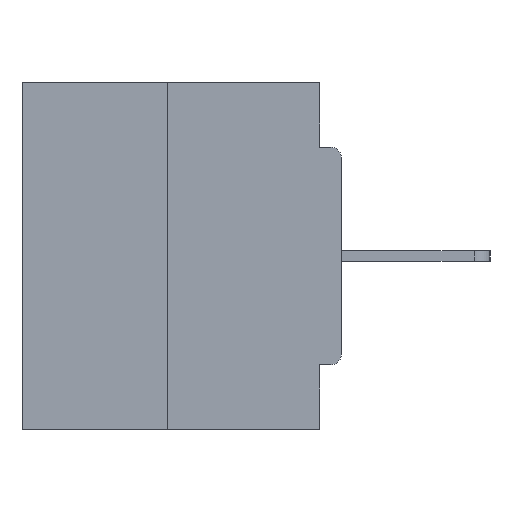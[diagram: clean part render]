
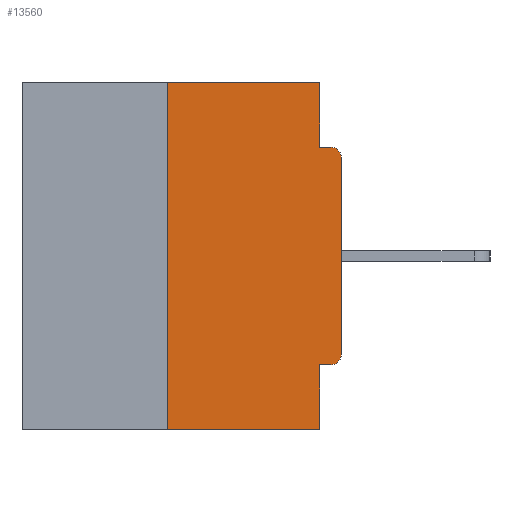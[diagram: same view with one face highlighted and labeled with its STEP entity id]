
A CAD part, left-side view. The second image highlights one B-rep face of the part: STEP entity #13560.
In plain terms, the highlighted planar face has unit normal (-1, 0, 0).
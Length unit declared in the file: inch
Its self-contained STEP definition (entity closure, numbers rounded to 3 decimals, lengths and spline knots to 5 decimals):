
#351 = EDGE_CURVE ( 'NONE', #19946, #1545, #28902, .T. ) ;
#399 = AXIS2_PLACEMENT_3D ( 'NONE', #8657, #17808, #10980 ) ;
#651 = LINE ( 'NONE', #26671, #6100 ) ;
#887 = VECTOR ( 'NONE', #17374, 39.37008 ) ;
#1545 = VERTEX_POINT ( 'NONE', #16060 ) ;
#1696 = AXIS2_PLACEMENT_3D ( 'NONE', #14558, #9563, #14642 ) ;
#1831 = VERTEX_POINT ( 'NONE', #20612 ) ;
#1855 = VERTEX_POINT ( 'NONE', #7345 ) ;
#2134 = CARTESIAN_POINT ( 'NONE',  ( 0., 0.46, 0. ) ) ;
#2260 = ORIENTED_EDGE ( 'NONE', *, *, #26404, .F. ) ;
#2754 = CIRCLE ( 'NONE', #399, 0.015 ) ;
#2787 = VERTEX_POINT ( 'NONE', #12997 ) ;
#3079 = LINE ( 'NONE', #26126, #11424 ) ;
#3674 = DIRECTION ( 'NONE',  ( 0., 0., -1. ) ) ;
#4083 = EDGE_CURVE ( 'NONE', #1855, #2787, #651, .T. ) ;
#4960 = VECTOR ( 'NONE', #9685, 39.37008 ) ;
#5619 = EDGE_CURVE ( 'NONE', #1831, #19946, #8171, .T. ) ;
#5686 = CARTESIAN_POINT ( 'NONE',  ( 0., 0.015, -0.0935 ) ) ;
#6100 = VECTOR ( 'NONE', #24642, 39.37008 ) ;
#6705 = LINE ( 'NONE', #8227, #27568 ) ;
#7345 = CARTESIAN_POINT ( 'NONE',  ( 0., 0., -0.3915 ) ) ;
#7649 = DIRECTION ( 'NONE',  ( 0., 0., -1. ) ) ;
#7907 = VERTEX_POINT ( 'NONE', #17746 ) ;
#7936 = AXIS2_PLACEMENT_3D ( 'NONE', #21834, #8075, #17742 ) ;
#8075 = DIRECTION ( 'NONE',  ( -1., 0., 0. ) ) ;
#8171 = LINE ( 'NONE', #25965, #4960 ) ;
#8227 = CARTESIAN_POINT ( 'NONE',  ( 0., 0.031, 0. ) ) ;
#8627 = ORIENTED_EDGE ( 'NONE', *, *, #17073, .T. ) ;
#8657 = CARTESIAN_POINT ( 'NONE',  ( 0., 0.015, -0.3915 ) ) ;
#9251 = LINE ( 'NONE', #20959, #17559 ) ;
#9563 = DIRECTION ( 'NONE',  ( 1., 0., 0. ) ) ;
#9685 = DIRECTION ( 'NONE',  ( 0., 0., 1. ) ) ;
#10751 = CARTESIAN_POINT ( 'NONE',  ( 0., 0., -0.0935 ) ) ;
#10980 = DIRECTION ( 'NONE',  ( 0., 0., -1. ) ) ;
#11026 = VERTEX_POINT ( 'NONE', #22522 ) ;
#11259 = ORIENTED_EDGE ( 'NONE', *, *, #15847, .T. ) ;
#11424 = VECTOR ( 'NONE', #7649, 39.37008 ) ;
#12436 = CARTESIAN_POINT ( 'NONE',  ( 0., 0.25, 0. ) ) ;
#12734 = EDGE_CURVE ( 'NONE', #22730, #25406, #3079, .T. ) ;
#12776 = CIRCLE ( 'NONE', #7936, 0.015 ) ;
#12997 = CARTESIAN_POINT ( 'NONE',  ( 0., 0., -0.1085 ) ) ;
#13276 = CARTESIAN_POINT ( 'NONE',  ( 0., 0.46, -0.5 ) ) ;
#13560 = ADVANCED_FACE ( 'NONE', ( #21498 ), #23352, .F. ) ;
#13973 = LINE ( 'NONE', #10751, #887 ) ;
#14558 = CARTESIAN_POINT ( 'NONE',  ( 0., 0.46, 0. ) ) ;
#14642 = DIRECTION ( 'NONE',  ( 0., 0., -1. ) ) ;
#15584 = ORIENTED_EDGE ( 'NONE', *, *, #16656, .F. ) ;
#15629 = VECTOR ( 'NONE', #20838, 39.37008 ) ;
#15659 = ORIENTED_EDGE ( 'NONE', *, *, #351, .F. ) ;
#15847 = EDGE_CURVE ( 'NONE', #2787, #19102, #12776, .T. ) ;
#15970 = ORIENTED_EDGE ( 'NONE', *, *, #19710, .T. ) ;
#16060 = CARTESIAN_POINT ( 'NONE',  ( 0., 0.031, 0. ) ) ;
#16089 = DIRECTION ( 'NONE',  ( 0., 1., 0. ) ) ;
#16656 = EDGE_CURVE ( 'NONE', #7907, #22730, #9251, .T. ) ;
#17073 = EDGE_CURVE ( 'NONE', #7907, #1855, #2754, .T. ) ;
#17374 = DIRECTION ( 'NONE',  ( 0., -1., 0. ) ) ;
#17559 = VECTOR ( 'NONE', #16089, 39.37008 ) ;
#17742 = DIRECTION ( 'NONE',  ( 0., 0., -1. ) ) ;
#17746 = CARTESIAN_POINT ( 'NONE',  ( 0., 0.015, -0.4065 ) ) ;
#17808 = DIRECTION ( 'NONE',  ( -1., 0., 0. ) ) ;
#18567 = ORIENTED_EDGE ( 'NONE', *, *, #5619, .F. ) ;
#19102 = VERTEX_POINT ( 'NONE', #5686 ) ;
#19542 = ORIENTED_EDGE ( 'NONE', *, *, #12734, .F. ) ;
#19710 = EDGE_CURVE ( 'NONE', #1831, #25406, #27354, .T. ) ;
#19946 = VERTEX_POINT ( 'NONE', #12436 ) ;
#20286 = CARTESIAN_POINT ( 'NONE',  ( 0., 0.031, -0.4065 ) ) ;
#20612 = CARTESIAN_POINT ( 'NONE',  ( 0., 0.25, -0.5 ) ) ;
#20838 = DIRECTION ( 'NONE',  ( 0., -1., 0. ) ) ;
#20959 = CARTESIAN_POINT ( 'NONE',  ( 0., 0., -0.4065 ) ) ;
#21498 = FACE_OUTER_BOUND ( 'NONE', #22801, .T. ) ;
#21579 = ORIENTED_EDGE ( 'NONE', *, *, #23057, .F. ) ;
#21834 = CARTESIAN_POINT ( 'NONE',  ( 0., 0.015, -0.1085 ) ) ;
#22522 = CARTESIAN_POINT ( 'NONE',  ( 0., 0.031, -0.0935 ) ) ;
#22730 = VERTEX_POINT ( 'NONE', #20286 ) ;
#22801 = EDGE_LOOP ( 'NONE', ( #15659, #18567, #15970, #19542, #15584, #8627, #27961, #11259, #21579, #2260 ) ) ;
#23057 = EDGE_CURVE ( 'NONE', #11026, #19102, #13973, .T. ) ;
#23352 = PLANE ( 'NONE',  #1696 ) ;
#24642 = DIRECTION ( 'NONE',  ( 0., 0., 1. ) ) ;
#25406 = VERTEX_POINT ( 'NONE', #27040 ) ;
#25965 = CARTESIAN_POINT ( 'NONE',  ( 0., 0.25, 0. ) ) ;
#26126 = CARTESIAN_POINT ( 'NONE',  ( 0., 0.031, -0.5 ) ) ;
#26404 = EDGE_CURVE ( 'NONE', #1545, #11026, #6705, .T. ) ;
#26671 = CARTESIAN_POINT ( 'NONE',  ( 0., 0., 0. ) ) ;
#27009 = DIRECTION ( 'NONE',  ( 0., -1., 0. ) ) ;
#27040 = CARTESIAN_POINT ( 'NONE',  ( 0., 0.031, -0.5 ) ) ;
#27354 = LINE ( 'NONE', #13276, #28795 ) ;
#27568 = VECTOR ( 'NONE', #3674, 39.37008 ) ;
#27961 = ORIENTED_EDGE ( 'NONE', *, *, #4083, .T. ) ;
#28795 = VECTOR ( 'NONE', #27009, 39.37008 ) ;
#28902 = LINE ( 'NONE', #2134, #15629 ) ;
